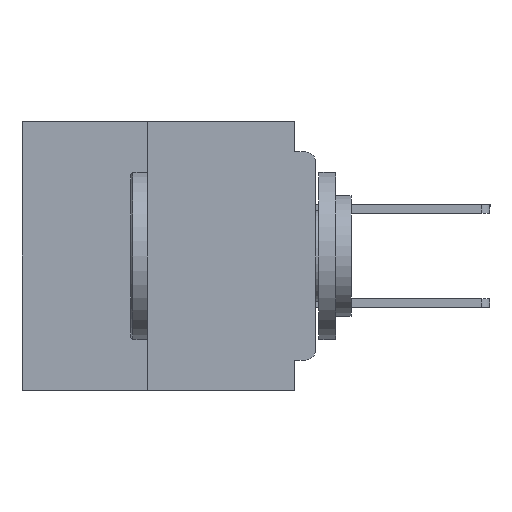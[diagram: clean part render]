
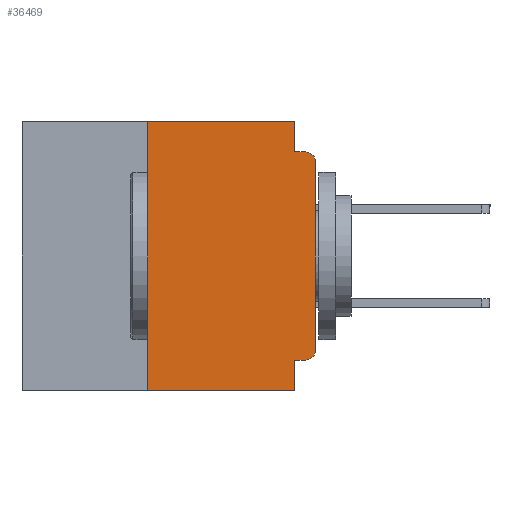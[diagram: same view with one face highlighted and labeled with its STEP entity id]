
A CAD part, left-side view. The second image highlights one B-rep face of the part: STEP entity #36469.
In plain terms, the highlighted planar face has unit normal (-1, 0, 0).
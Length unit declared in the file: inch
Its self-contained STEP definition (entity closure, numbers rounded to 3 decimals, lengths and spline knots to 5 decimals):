
#164 = EDGE_CURVE ( 'NONE', #17585, #25837, #24186, .T. ) ;
#701 = DIRECTION ( 'NONE',  ( 0., 0., 1. ) ) ;
#1208 = EDGE_CURVE ( 'NONE', #25837, #11025, #14324, .T. ) ;
#1403 = CARTESIAN_POINT ( 'NONE',  ( 0., 0., -0.34 ) ) ;
#2832 = VECTOR ( 'NONE', #20660, 39.37008 ) ;
#3190 = VECTOR ( 'NONE', #35748, 39.37008 ) ;
#3654 = VERTEX_POINT ( 'NONE', #1403 ) ;
#4134 = CARTESIAN_POINT ( 'NONE',  ( 0., 0.25, -0.4 ) ) ;
#4891 = VERTEX_POINT ( 'NONE', #31962 ) ;
#5773 = LINE ( 'NONE', #9046, #14832 ) ;
#6172 = EDGE_CURVE ( 'NONE', #39936, #4891, #5773, .T. ) ;
#6700 = LINE ( 'NONE', #35174, #45094 ) ;
#7087 = VECTOR ( 'NONE', #37203, 39.37008 ) ;
#7521 = CARTESIAN_POINT ( 'NONE',  ( 0., 0.031, -0.4 ) ) ;
#8183 = CARTESIAN_POINT ( 'NONE',  ( 0., 0.015, -0.06 ) ) ;
#8198 = CARTESIAN_POINT ( 'NONE',  ( 0., 0.25, -0.4 ) ) ;
#8401 = PLANE ( 'NONE',  #8612 ) ;
#8612 = AXIS2_PLACEMENT_3D ( 'NONE', #35326, #12282, #39196 ) ;
#8769 = CIRCLE ( 'NONE', #25953, 0.015 ) ;
#8832 = CARTESIAN_POINT ( 'NONE',  ( 0., 0.437, -0.4 ) ) ;
#9046 = CARTESIAN_POINT ( 'NONE',  ( 0., 0., -0.045 ) ) ;
#9132 = EDGE_CURVE ( 'NONE', #11025, #39936, #34858, .T. ) ;
#10845 = EDGE_CURVE ( 'NONE', #18595, #3654, #8769, .T. ) ;
#11025 = VERTEX_POINT ( 'NONE', #11068 ) ;
#11068 = CARTESIAN_POINT ( 'NONE',  ( 0., 0.031, 0. ) ) ;
#11583 = CARTESIAN_POINT ( 'NONE',  ( 0., 0.031, -0.355 ) ) ;
#12068 = DIRECTION ( 'NONE',  ( 0., 0., -1. ) ) ;
#12282 = DIRECTION ( 'NONE',  ( 1., 0., 0. ) ) ;
#12824 = VECTOR ( 'NONE', #20479, 39.37008 ) ;
#12946 = EDGE_LOOP ( 'NONE', ( #37333, #22845, #17511, #32515, #19860, #26910, #37053, #28930, #19076, #33445 ) ) ;
#14108 = DIRECTION ( 'NONE',  ( -1., 0., 0. ) ) ;
#14324 = LINE ( 'NONE', #31749, #2832 ) ;
#14832 = VECTOR ( 'NONE', #20806, 39.37008 ) ;
#14871 = FACE_OUTER_BOUND ( 'NONE', #12946, .T. ) ;
#15819 = EDGE_CURVE ( 'NONE', #3654, #44145, #6700, .T. ) ;
#17511 = ORIENTED_EDGE ( 'NONE', *, *, #6172, .F. ) ;
#17585 = VERTEX_POINT ( 'NONE', #8198 ) ;
#18595 = VERTEX_POINT ( 'NONE', #37714 ) ;
#18646 = LINE ( 'NONE', #41057, #7087 ) ;
#19076 = ORIENTED_EDGE ( 'NONE', *, *, #38514, .F. ) ;
#19442 = CARTESIAN_POINT ( 'NONE',  ( 0., 0.031, 0. ) ) ;
#19860 = ORIENTED_EDGE ( 'NONE', *, *, #1208, .F. ) ;
#20117 = CARTESIAN_POINT ( 'NONE',  ( 0., 0.25, 0. ) ) ;
#20479 = DIRECTION ( 'NONE',  ( 0., 1., 0. ) ) ;
#20660 = DIRECTION ( 'NONE',  ( 0., -1., 0. ) ) ;
#20806 = DIRECTION ( 'NONE',  ( 0., -1., 0. ) ) ;
#21239 = EDGE_CURVE ( 'NONE', #32801, #32749, #18646, .T. ) ;
#22845 = ORIENTED_EDGE ( 'NONE', *, *, #32890, .T. ) ;
#23161 = LINE ( 'NONE', #24170, #12824 ) ;
#23297 = DIRECTION ( 'NONE',  ( 0., 0., -1. ) ) ;
#24170 = CARTESIAN_POINT ( 'NONE',  ( 0., 0., -0.355 ) ) ;
#24186 = LINE ( 'NONE', #4134, #31892 ) ;
#24732 = VECTOR ( 'NONE', #23297, 39.37008 ) ;
#25837 = VERTEX_POINT ( 'NONE', #20117 ) ;
#25953 = AXIS2_PLACEMENT_3D ( 'NONE', #37136, #14108, #40991 ) ;
#26386 = AXIS2_PLACEMENT_3D ( 'NONE', #8183, #35110, #12068 ) ;
#26910 = ORIENTED_EDGE ( 'NONE', *, *, #164, .F. ) ;
#28930 = ORIENTED_EDGE ( 'NONE', *, *, #21239, .F. ) ;
#31749 = CARTESIAN_POINT ( 'NONE',  ( 0., 0.437, 0. ) ) ;
#31892 = VECTOR ( 'NONE', #701, 39.37008 ) ;
#31962 = CARTESIAN_POINT ( 'NONE',  ( 0., 0.015, -0.045 ) ) ;
#32515 = ORIENTED_EDGE ( 'NONE', *, *, #9132, .F. ) ;
#32749 = VERTEX_POINT ( 'NONE', #7521 ) ;
#32801 = VERTEX_POINT ( 'NONE', #11583 ) ;
#32890 = EDGE_CURVE ( 'NONE', #44145, #4891, #38618, .T. ) ;
#33343 = CARTESIAN_POINT ( 'NONE',  ( 0., 0.031, -0.045 ) ) ;
#33445 = ORIENTED_EDGE ( 'NONE', *, *, #10845, .T. ) ;
#34858 = LINE ( 'NONE', #19442, #24732 ) ;
#35110 = DIRECTION ( 'NONE',  ( -1., 0., 0. ) ) ;
#35174 = CARTESIAN_POINT ( 'NONE',  ( 0., 0., 0. ) ) ;
#35326 = CARTESIAN_POINT ( 'NONE',  ( 0., 0.437, 0. ) ) ;
#35748 = DIRECTION ( 'NONE',  ( 0., -1., 0. ) ) ;
#36469 = ADVANCED_FACE ( 'NONE', ( #14871 ), #8401, .F. ) ;
#37053 = ORIENTED_EDGE ( 'NONE', *, *, #41235, .T. ) ;
#37136 = CARTESIAN_POINT ( 'NONE',  ( 0., 0.015, -0.34 ) ) ;
#37203 = DIRECTION ( 'NONE',  ( 0., 0., -1. ) ) ;
#37333 = ORIENTED_EDGE ( 'NONE', *, *, #15819, .T. ) ;
#37714 = CARTESIAN_POINT ( 'NONE',  ( 0., 0.015, -0.355 ) ) ;
#38514 = EDGE_CURVE ( 'NONE', #18595, #32801, #23161, .T. ) ;
#38618 = CIRCLE ( 'NONE', #26386, 0.015 ) ;
#39050 = DIRECTION ( 'NONE',  ( 0., 0., 1. ) ) ;
#39196 = DIRECTION ( 'NONE',  ( 0., 0., -1. ) ) ;
#39936 = VERTEX_POINT ( 'NONE', #33343 ) ;
#40991 = DIRECTION ( 'NONE',  ( 0., 0., -1. ) ) ;
#41057 = CARTESIAN_POINT ( 'NONE',  ( 0., 0.031, -0.4 ) ) ;
#41235 = EDGE_CURVE ( 'NONE', #17585, #32749, #42880, .T. ) ;
#42880 = LINE ( 'NONE', #8832, #3190 ) ;
#44145 = VERTEX_POINT ( 'NONE', #45576 ) ;
#45094 = VECTOR ( 'NONE', #39050, 39.37008 ) ;
#45576 = CARTESIAN_POINT ( 'NONE',  ( 0., 0., -0.06 ) ) ;
